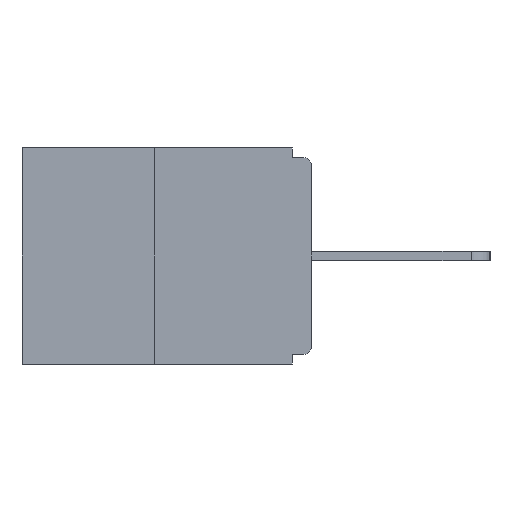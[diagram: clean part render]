
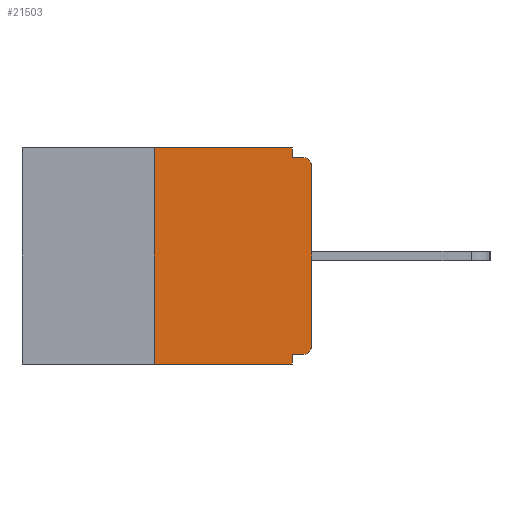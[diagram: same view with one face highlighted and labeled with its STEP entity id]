
A CAD part, left-side view. The second image highlights one B-rep face of the part: STEP entity #21503.
In plain terms, the highlighted planar face has unit normal (-1, 0, 0).
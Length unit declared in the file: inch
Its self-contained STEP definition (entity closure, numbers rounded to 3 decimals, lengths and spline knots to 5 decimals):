
#85 = CARTESIAN_POINT ( 'NONE',  ( 0., 0.031, -0.343 ) ) ;
#437 = CARTESIAN_POINT ( 'NONE',  ( 0., 0.25, 0. ) ) ;
#805 = DIRECTION ( 'NONE',  ( 0., 1., 0. ) ) ;
#890 = VECTOR ( 'NONE', #6954, 39.37008 ) ;
#1161 = VECTOR ( 'NONE', #18871, 39.37008 ) ;
#1255 = AXIS2_PLACEMENT_3D ( 'NONE', #6343, #20853, #18820 ) ;
#1278 = CARTESIAN_POINT ( 'NONE',  ( 0., 0., 0. ) ) ;
#1419 = VERTEX_POINT ( 'NONE', #8660 ) ;
#1903 = ORIENTED_EDGE ( 'NONE', *, *, #15302, .F. ) ;
#1939 = VERTEX_POINT ( 'NONE', #23497 ) ;
#1970 = DIRECTION ( 'NONE',  ( 1., 0., 0. ) ) ;
#1997 = DIRECTION ( 'NONE',  ( 0., 0., -1. ) ) ;
#2250 = CARTESIAN_POINT ( 'NONE',  ( 0., 0.031, -0.015 ) ) ;
#2262 = CARTESIAN_POINT ( 'NONE',  ( 0., 0.031, -0.328 ) ) ;
#2322 = DIRECTION ( 'NONE',  ( 0., 0., -1. ) ) ;
#3255 = AXIS2_PLACEMENT_3D ( 'NONE', #19998, #14700, #1997 ) ;
#3890 = DIRECTION ( 'NONE',  ( 0., -1., 0. ) ) ;
#4488 = LINE ( 'NONE', #4614, #1161 ) ;
#4614 = CARTESIAN_POINT ( 'NONE',  ( 0., 0., -0.015 ) ) ;
#4766 = CARTESIAN_POINT ( 'NONE',  ( 0., 0., -0.328 ) ) ;
#4807 = VERTEX_POINT ( 'NONE', #19783 ) ;
#5616 = EDGE_CURVE ( 'NONE', #6602, #8309, #10165, .T. ) ;
#5751 = VECTOR ( 'NONE', #3890, 39.37008 ) ;
#5935 = EDGE_LOOP ( 'NONE', ( #23270, #20250, #18863, #1903, #11875, #14082, #10990, #20195, #8040, #6635 ) ) ;
#6275 = CARTESIAN_POINT ( 'NONE',  ( 0., 0.031, -0.343 ) ) ;
#6343 = CARTESIAN_POINT ( 'NONE',  ( 0., 0.015, -0.03 ) ) ;
#6602 = VERTEX_POINT ( 'NONE', #10902 ) ;
#6635 = ORIENTED_EDGE ( 'NONE', *, *, #5616, .F. ) ;
#6819 = CARTESIAN_POINT ( 'NONE',  ( 0., 0.015, -0.015 ) ) ;
#6954 = DIRECTION ( 'NONE',  ( 0., -1., 0. ) ) ;
#6968 = VERTEX_POINT ( 'NONE', #19661 ) ;
#8040 = ORIENTED_EDGE ( 'NONE', *, *, #21681, .F. ) ;
#8253 = DIRECTION ( 'NONE',  ( 0., 0., -1. ) ) ;
#8309 = VERTEX_POINT ( 'NONE', #2250 ) ;
#8660 = CARTESIAN_POINT ( 'NONE',  ( 0., 0.25, -0.343 ) ) ;
#8755 = LINE ( 'NONE', #16084, #890 ) ;
#9157 = VECTOR ( 'NONE', #805, 39.37008 ) ;
#10149 = CIRCLE ( 'NONE', #3255, 0.015 ) ;
#10165 = LINE ( 'NONE', #22532, #15137 ) ;
#10379 = LINE ( 'NONE', #1278, #22993 ) ;
#10902 = CARTESIAN_POINT ( 'NONE',  ( 0., 0.031, 0. ) ) ;
#10990 = ORIENTED_EDGE ( 'NONE', *, *, #19792, .T. ) ;
#11071 = CARTESIAN_POINT ( 'NONE',  ( 0., 0.46, 0. ) ) ;
#11176 = PLANE ( 'NONE',  #15324 ) ;
#11875 = ORIENTED_EDGE ( 'NONE', *, *, #19601, .F. ) ;
#13088 = FACE_OUTER_BOUND ( 'NONE', #5935, .T. ) ;
#13520 = VERTEX_POINT ( 'NONE', #17272 ) ;
#14082 = ORIENTED_EDGE ( 'NONE', *, *, #15326, .T. ) ;
#14559 = CARTESIAN_POINT ( 'NONE',  ( 0., 0.46, -0.343 ) ) ;
#14588 = DIRECTION ( 'NONE',  ( 0., 0., -1. ) ) ;
#14699 = DIRECTION ( 'NONE',  ( 0., 0., 1. ) ) ;
#14700 = DIRECTION ( 'NONE',  ( -1., 0., 0. ) ) ;
#14822 = LINE ( 'NONE', #85, #21646 ) ;
#15017 = VERTEX_POINT ( 'NONE', #2262 ) ;
#15137 = VECTOR ( 'NONE', #8253, 39.37008 ) ;
#15302 = EDGE_CURVE ( 'NONE', #15017, #21781, #14822, .T. ) ;
#15324 = AXIS2_PLACEMENT_3D ( 'NONE', #11071, #1970, #2322 ) ;
#15326 = EDGE_CURVE ( 'NONE', #6968, #1939, #10149, .T. ) ;
#15906 = DIRECTION ( 'NONE',  ( 0., 0., 1. ) ) ;
#16084 = CARTESIAN_POINT ( 'NONE',  ( 0., 0.46, 0. ) ) ;
#17272 = CARTESIAN_POINT ( 'NONE',  ( 0., 0.25, 0. ) ) ;
#18375 = VECTOR ( 'NONE', #14699, 39.37008 ) ;
#18820 = DIRECTION ( 'NONE',  ( 0., 0., -1. ) ) ;
#18863 = ORIENTED_EDGE ( 'NONE', *, *, #21614, .T. ) ;
#18871 = DIRECTION ( 'NONE',  ( 0., -1., 0. ) ) ;
#19304 = VERTEX_POINT ( 'NONE', #6819 ) ;
#19601 = EDGE_CURVE ( 'NONE', #6968, #15017, #20829, .T. ) ;
#19661 = CARTESIAN_POINT ( 'NONE',  ( 0., 0.015, -0.328 ) ) ;
#19783 = CARTESIAN_POINT ( 'NONE',  ( 0., 0., -0.03 ) ) ;
#19792 = EDGE_CURVE ( 'NONE', #1939, #4807, #10379, .T. ) ;
#19998 = CARTESIAN_POINT ( 'NONE',  ( 0., 0.015, -0.313 ) ) ;
#20195 = ORIENTED_EDGE ( 'NONE', *, *, #22642, .T. ) ;
#20250 = ORIENTED_EDGE ( 'NONE', *, *, #21137, .F. ) ;
#20594 = LINE ( 'NONE', #437, #18375 ) ;
#20829 = LINE ( 'NONE', #4766, #9157 ) ;
#20853 = DIRECTION ( 'NONE',  ( -1., 0., 0. ) ) ;
#21137 = EDGE_CURVE ( 'NONE', #1419, #13520, #20594, .T. ) ;
#21182 = CIRCLE ( 'NONE', #1255, 0.015 ) ;
#21503 = ADVANCED_FACE ( 'NONE', ( #13088 ), #11176, .F. ) ;
#21614 = EDGE_CURVE ( 'NONE', #1419, #21781, #21994, .T. ) ;
#21646 = VECTOR ( 'NONE', #14588, 39.37008 ) ;
#21681 = EDGE_CURVE ( 'NONE', #8309, #19304, #4488, .T. ) ;
#21781 = VERTEX_POINT ( 'NONE', #6275 ) ;
#21994 = LINE ( 'NONE', #14559, #5751 ) ;
#22532 = CARTESIAN_POINT ( 'NONE',  ( 0., 0.031, 0. ) ) ;
#22642 = EDGE_CURVE ( 'NONE', #4807, #19304, #21182, .T. ) ;
#22993 = VECTOR ( 'NONE', #15906, 39.37008 ) ;
#23270 = ORIENTED_EDGE ( 'NONE', *, *, #23696, .F. ) ;
#23497 = CARTESIAN_POINT ( 'NONE',  ( 0., 0., -0.313 ) ) ;
#23696 = EDGE_CURVE ( 'NONE', #13520, #6602, #8755, .T. ) ;
